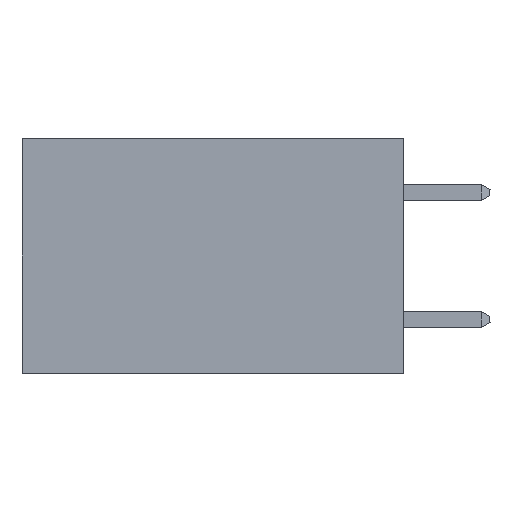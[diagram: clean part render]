
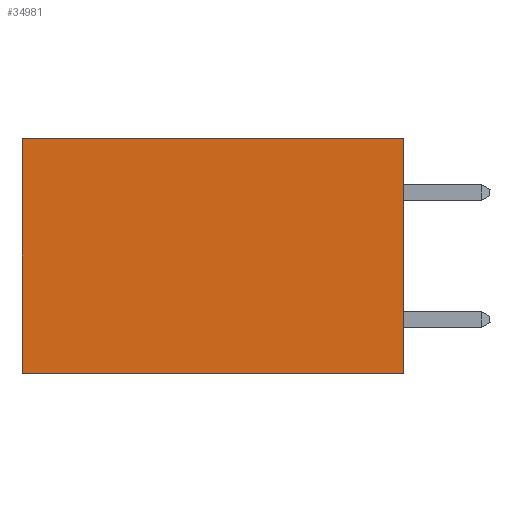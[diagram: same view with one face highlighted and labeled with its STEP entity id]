
A CAD part, left-side view. The second image highlights one B-rep face of the part: STEP entity #34981.
In plain terms, the highlighted planar face has unit normal (-1, 0, 0).
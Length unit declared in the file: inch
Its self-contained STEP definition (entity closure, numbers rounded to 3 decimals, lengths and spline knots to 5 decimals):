
#1126 = CARTESIAN_POINT ( 'NONE',  ( 0.2875, 0., 0. ) ) ;
#1702 = CARTESIAN_POINT ( 'NONE',  ( 0.2875, 0., 0. ) ) ;
#1981 = CARTESIAN_POINT ( 'NONE',  ( 0.2875, 0.6, 0. ) ) ;
#3226 = DIRECTION ( 'NONE',  ( 0., 1., 0. ) ) ;
#3522 = DIRECTION ( 'NONE',  ( 0., 1., 0. ) ) ;
#3756 = VERTEX_POINT ( 'NONE', #1981 ) ;
#5272 = VECTOR ( 'NONE', #19168, 39.37008 ) ;
#8709 = CARTESIAN_POINT ( 'NONE',  ( 0.2875, 0.6, -0.37 ) ) ;
#8930 = PLANE ( 'NONE',  #35350 ) ;
#10677 = ORIENTED_EDGE ( 'NONE', *, *, #24242, .F. ) ;
#12604 = DIRECTION ( 'NONE',  ( 0., 0., -1. ) ) ;
#13630 = EDGE_CURVE ( 'NONE', #29466, #3756, #25251, .T. ) ;
#14074 = EDGE_LOOP ( 'NONE', ( #43945, #33072, #10677, #27795 ) ) ;
#15538 = VECTOR ( 'NONE', #3226, 39.37008 ) ;
#15968 = EDGE_CURVE ( 'NONE', #3756, #23750, #38658, .T. ) ;
#19168 = DIRECTION ( 'NONE',  ( 0., 0., -1. ) ) ;
#22078 = FACE_OUTER_BOUND ( 'NONE', #14074, .T. ) ;
#23750 = VERTEX_POINT ( 'NONE', #8709 ) ;
#24242 = EDGE_CURVE ( 'NONE', #29466, #42350, #42786, .T. ) ;
#24847 = CARTESIAN_POINT ( 'NONE',  ( 0.2875, 0., 0. ) ) ;
#24973 = CARTESIAN_POINT ( 'NONE',  ( 0.2875, 0., -0.37 ) ) ;
#25251 = LINE ( 'NONE', #24847, #15538 ) ;
#26882 = EDGE_CURVE ( 'NONE', #42350, #23750, #34667, .T. ) ;
#27795 = ORIENTED_EDGE ( 'NONE', *, *, #13630, .T. ) ;
#28993 = VECTOR ( 'NONE', #37794, 39.37008 ) ;
#29466 = VERTEX_POINT ( 'NONE', #30436 ) ;
#30436 = CARTESIAN_POINT ( 'NONE',  ( 0.2875, 0., 0. ) ) ;
#33072 = ORIENTED_EDGE ( 'NONE', *, *, #26882, .F. ) ;
#34146 = CARTESIAN_POINT ( 'NONE',  ( 0.2875, 0.6, 0. ) ) ;
#34426 = DIRECTION ( 'NONE',  ( 1., 0., 0. ) ) ;
#34667 = LINE ( 'NONE', #43372, #35831 ) ;
#34981 = ADVANCED_FACE ( 'NONE', ( #22078 ), #8930, .F. ) ;
#35350 = AXIS2_PLACEMENT_3D ( 'NONE', #1702, #34426, #12604 ) ;
#35831 = VECTOR ( 'NONE', #3522, 39.37008 ) ;
#37794 = DIRECTION ( 'NONE',  ( 0., 0., -1. ) ) ;
#38658 = LINE ( 'NONE', #34146, #28993 ) ;
#42350 = VERTEX_POINT ( 'NONE', #24973 ) ;
#42786 = LINE ( 'NONE', #1126, #5272 ) ;
#43372 = CARTESIAN_POINT ( 'NONE',  ( 0.2875, 0., -0.37 ) ) ;
#43945 = ORIENTED_EDGE ( 'NONE', *, *, #15968, .T. ) ;
